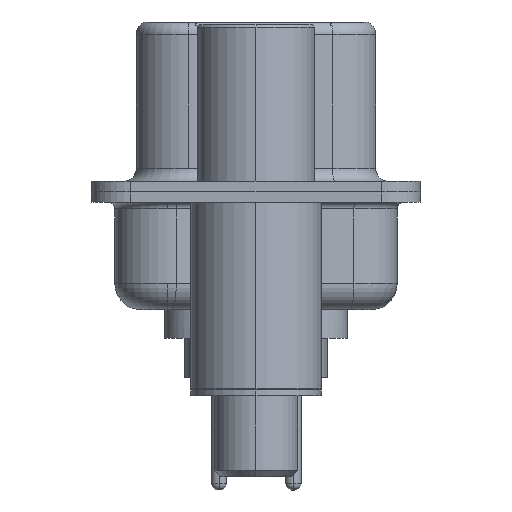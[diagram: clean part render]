
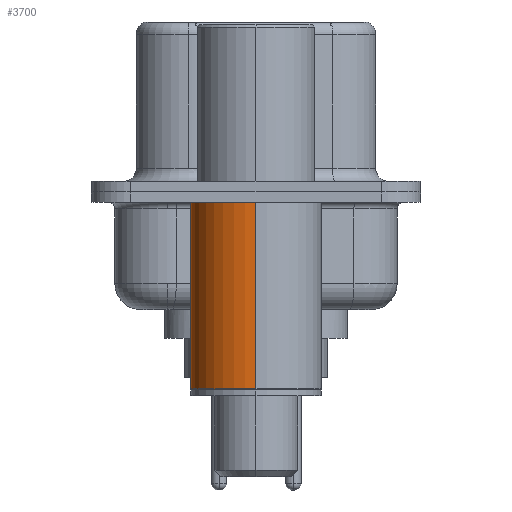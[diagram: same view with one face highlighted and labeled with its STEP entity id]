
A CAD part, left-side view. The second image highlights one B-rep face of the part: STEP entity #3700.
In plain terms, the highlighted cylindrical face has radius 2.5 mm (diameter 5 mm), a partial arc.
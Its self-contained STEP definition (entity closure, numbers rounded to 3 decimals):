
#10 = EDGE_LOOP ( 'NONE', ( #5260, #22436, #24832, #10410 ) ) ;
#570 = VERTEX_POINT ( 'NONE', #6010 ) ;
#884 = DIRECTION ( 'NONE',  ( 0., 0., 1. ) ) ;
#2726 = CIRCLE ( 'NONE', #16317, 2.5 ) ;
#3638 = DIRECTION ( 'NONE',  ( 0., 0., 1. ) ) ;
#3700 = ADVANCED_FACE ( 'NONE', ( #9546 ), #8919, .T. ) ;
#3911 = EDGE_CURVE ( 'NONE', #11638, #21279, #21414, .T. ) ;
#4264 = CARTESIAN_POINT ( 'NONE',  ( 2.5, 0., -7.525 ) ) ;
#4481 = VERTEX_POINT ( 'NONE', #4264 ) ;
#4756 = DIRECTION ( 'NONE',  ( 0., 0., 1. ) ) ;
#5260 = ORIENTED_EDGE ( 'NONE', *, *, #7914, .T. ) ;
#5786 = LINE ( 'NONE', #9945, #10480 ) ;
#6010 = CARTESIAN_POINT ( 'NONE',  ( 2.5, 0., -0.4 ) ) ;
#6097 = DIRECTION ( 'NONE',  ( 0., 0., 1. ) ) ;
#6921 = CARTESIAN_POINT ( 'NONE',  ( -2.5, 0., 0.581 ) ) ;
#7068 = EDGE_CURVE ( 'NONE', #570, #21279, #2726, .T. ) ;
#7914 = EDGE_CURVE ( 'NONE', #4481, #11638, #17946, .T. ) ;
#8919 = CYLINDRICAL_SURFACE ( 'NONE', #21190, 2.5 ) ;
#9546 = FACE_OUTER_BOUND ( 'NONE', #10, .T. ) ;
#9945 = CARTESIAN_POINT ( 'NONE',  ( 2.5, 0., 0.581 ) ) ;
#10410 = ORIENTED_EDGE ( 'NONE', *, *, #19904, .F. ) ;
#10476 = VECTOR ( 'NONE', #884, 1000. ) ;
#10480 = VECTOR ( 'NONE', #6097, 1000. ) ;
#11638 = VERTEX_POINT ( 'NONE', #14121 ) ;
#11993 = DIRECTION ( 'NONE',  ( 1., 0., 0. ) ) ;
#14121 = CARTESIAN_POINT ( 'NONE',  ( -2.5, 0., -7.525 ) ) ;
#15774 = CARTESIAN_POINT ( 'NONE',  ( 0., 0., -7.525 ) ) ;
#16153 = CARTESIAN_POINT ( 'NONE',  ( 0., 0., 0.581 ) ) ;
#16317 = AXIS2_PLACEMENT_3D ( 'NONE', #16936, #4756, #18997 ) ;
#16936 = CARTESIAN_POINT ( 'NONE',  ( 0., 0., -0.4 ) ) ;
#17869 = DIRECTION ( 'NONE',  ( 1., 0., 0. ) ) ;
#17946 = CIRCLE ( 'NONE', #25692, 2.5 ) ;
#18997 = DIRECTION ( 'NONE',  ( 1., 0., 0. ) ) ;
#19904 = EDGE_CURVE ( 'NONE', #4481, #570, #5786, .T. ) ;
#20276 = DIRECTION ( 'NONE',  ( 0., 0., 1. ) ) ;
#21190 = AXIS2_PLACEMENT_3D ( 'NONE', #16153, #20276, #11993 ) ;
#21279 = VERTEX_POINT ( 'NONE', #24436 ) ;
#21414 = LINE ( 'NONE', #6921, #10476 ) ;
#22436 = ORIENTED_EDGE ( 'NONE', *, *, #3911, .T. ) ;
#24436 = CARTESIAN_POINT ( 'NONE',  ( -2.5, 0., -0.4 ) ) ;
#24832 = ORIENTED_EDGE ( 'NONE', *, *, #7068, .F. ) ;
#25692 = AXIS2_PLACEMENT_3D ( 'NONE', #15774, #3638, #17869 ) ;
